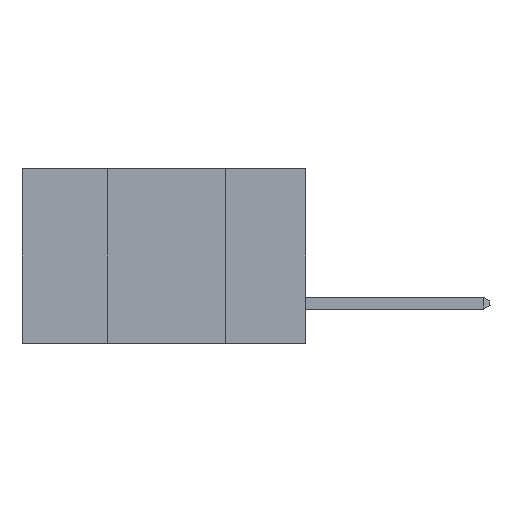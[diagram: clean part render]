
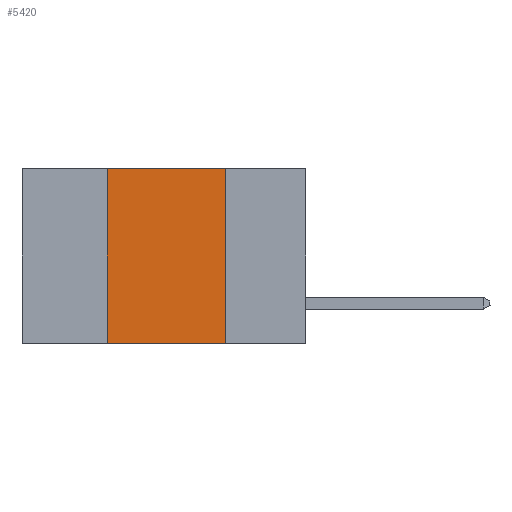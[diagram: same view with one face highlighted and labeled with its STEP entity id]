
A CAD part, left-side view. The second image highlights one B-rep face of the part: STEP entity #5420.
In plain terms, the highlighted planar face has unit normal (-1, 0, 0).
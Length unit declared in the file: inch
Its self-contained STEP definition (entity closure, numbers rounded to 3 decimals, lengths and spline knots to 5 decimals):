
#610 = PLANE ( 'NONE',  #5005 ) ;
#681 = ORIENTED_EDGE ( 'NONE', *, *, #5642, .F. ) ;
#873 = CARTESIAN_POINT ( 'NONE',  ( 0., 0.42, 0. ) ) ;
#1296 = CARTESIAN_POINT ( 'NONE',  ( 0., 0.6, 0. ) ) ;
#1324 = EDGE_LOOP ( 'NONE', ( #681, #2216, #9110, #5367 ) ) ;
#1508 = EDGE_CURVE ( 'NONE', #7927, #3549, #4430, .T. ) ;
#2216 = ORIENTED_EDGE ( 'NONE', *, *, #4624, .F. ) ;
#2217 = CARTESIAN_POINT ( 'NONE',  ( 0., 0.6, -0.37 ) ) ;
#2986 = VECTOR ( 'NONE', #5615, 39.37008 ) ;
#2993 = DIRECTION ( 'NONE',  ( 0., 0., -1. ) ) ;
#3519 = FACE_OUTER_BOUND ( 'NONE', #1324, .T. ) ;
#3531 = EDGE_CURVE ( 'NONE', #7927, #5151, #9470, .T. ) ;
#3549 = VERTEX_POINT ( 'NONE', #4770 ) ;
#3876 = DIRECTION ( 'NONE',  ( 0., -1., 0. ) ) ;
#4317 = DIRECTION ( 'NONE',  ( 0., -1., 0. ) ) ;
#4430 = LINE ( 'NONE', #2217, #10396 ) ;
#4624 = EDGE_CURVE ( 'NONE', #5151, #9598, #8285, .T. ) ;
#4726 = CARTESIAN_POINT ( 'NONE',  ( 0., 0.42, 0. ) ) ;
#4770 = CARTESIAN_POINT ( 'NONE',  ( 0., 0.17, -0.37 ) ) ;
#5005 = AXIS2_PLACEMENT_3D ( 'NONE', #1296, #10194, #2993 ) ;
#5151 = VERTEX_POINT ( 'NONE', #4726 ) ;
#5367 = ORIENTED_EDGE ( 'NONE', *, *, #1508, .T. ) ;
#5420 = ADVANCED_FACE ( 'NONE', ( #3519 ), #610, .F. ) ;
#5615 = DIRECTION ( 'NONE',  ( 0., 0., 1. ) ) ;
#5642 = EDGE_CURVE ( 'NONE', #9598, #3549, #8601, .T. ) ;
#7129 = DIRECTION ( 'NONE',  ( 0., 0., -1. ) ) ;
#7927 = VERTEX_POINT ( 'NONE', #9605 ) ;
#8285 = LINE ( 'NONE', #8961, #10067 ) ;
#8601 = LINE ( 'NONE', #9622, #10382 ) ;
#8961 = CARTESIAN_POINT ( 'NONE',  ( 0., 0.6, 0. ) ) ;
#9110 = ORIENTED_EDGE ( 'NONE', *, *, #3531, .F. ) ;
#9238 = CARTESIAN_POINT ( 'NONE',  ( 0., 0.17, 0. ) ) ;
#9470 = LINE ( 'NONE', #873, #2986 ) ;
#9598 = VERTEX_POINT ( 'NONE', #9238 ) ;
#9605 = CARTESIAN_POINT ( 'NONE',  ( 0., 0.42, -0.37 ) ) ;
#9622 = CARTESIAN_POINT ( 'NONE',  ( 0., 0.17, 0. ) ) ;
#10067 = VECTOR ( 'NONE', #4317, 39.37008 ) ;
#10194 = DIRECTION ( 'NONE',  ( 1., 0., 0. ) ) ;
#10382 = VECTOR ( 'NONE', #7129, 39.37008 ) ;
#10396 = VECTOR ( 'NONE', #3876, 39.37008 ) ;
